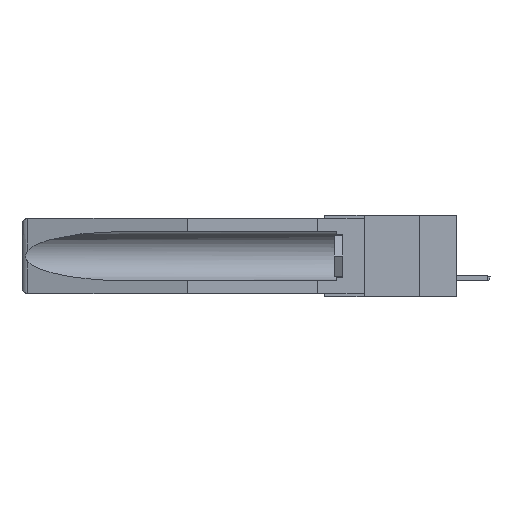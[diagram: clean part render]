
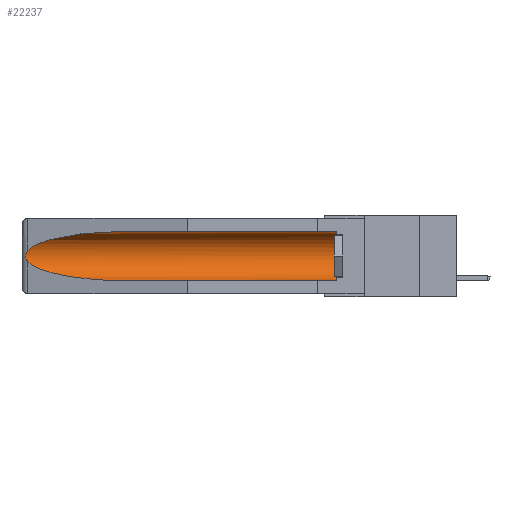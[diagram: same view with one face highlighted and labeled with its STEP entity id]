
A CAD part, left-side view. The second image highlights one B-rep face of the part: STEP entity #22237.
In plain terms, the highlighted cylindrical face has radius 2.857 mm (diameter 5.715 mm), a partial arc.
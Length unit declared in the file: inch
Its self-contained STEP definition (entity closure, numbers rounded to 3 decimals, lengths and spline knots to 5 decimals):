
#723 = CARTESIAN_POINT ( 'NONE',  ( 0.26654, 1.53092, -0.15636 ) ) ;
#850 = ORIENTED_EDGE ( 'NONE', *, *, #21930, .T. ) ;
#1276 = CARTESIAN_POINT ( 'NONE',  ( 0.26597, 1.5296, -0.19026 ) ) ;
#1510 = FACE_OUTER_BOUND ( 'NONE', #3524, .T. ) ;
#1536 = VECTOR ( 'NONE', #4677, 39.37008 ) ;
#1788 = CARTESIAN_POINT ( 'NONE',  ( 0.2675, 1.53308, -0.17534 ) ) ;
#2054 = LINE ( 'NONE', #13014, #4106 ) ;
#3070 = B_SPLINE_CURVE_WITH_KNOTS ( 'NONE', 3,
 ( #3275, #9907, #723, #17129, #3477, #1788, #18815, #14418, #1276, #5667 ),
 .UNSPECIFIED., .F., .F.,
 ( 4, 2, 2, 2, 4 ),
 ( 0., 0.00029, 0.00058, 0.00087, 0.00117 ),
 .UNSPECIFIED. ) ;
#3275 = CARTESIAN_POINT ( 'NONE',  ( 0.26537, 1.52718, -0.14972 ) ) ;
#3477 = CARTESIAN_POINT ( 'NONE',  ( 0.2675, 1.53308, -0.16763 ) ) ;
#3524 = EDGE_LOOP ( 'NONE', ( #13509, #11887, #20888, #19044, #21107, #850 ) ) ;
#4014 = CARTESIAN_POINT ( 'NONE',  ( 0.155, 1.07973, -0.059 ) ) ;
#4043 = VERTEX_POINT ( 'NONE', #14770 ) ;
#4106 = VECTOR ( 'NONE', #6475, 39.37008 ) ;
#4454 = CARTESIAN_POINT ( 'NONE',  ( 0.25451, 1.48313, -0.24835 ) ) ;
#4677 = DIRECTION ( 'NONE',  ( 0., 1., 0. ) ) ;
#5005 =( BOUNDED_CURVE ( )  B_SPLINE_CURVE ( 3, ( #15228, #4454, #21779, #19602 ),
 .UNSPECIFIED., .F., .F. ) 
 B_SPLINE_CURVE_WITH_KNOTS ( ( 4, 4 ),
 ( 0.1948, 1.5708 ),
 .UNSPECIFIED. ) 
 CURVE ( )  GEOMETRIC_REPRESENTATION_ITEM ( )  RATIONAL_B_SPLINE_CURVE ( ( 1., 0.848, 0.848, 1. ) ) 
 REPRESENTATION_ITEM ( '' )  );
#5667 = CARTESIAN_POINT ( 'NONE',  ( 0.26537, 1.52718, -0.19328 ) ) ;
#6019 = CARTESIAN_POINT ( 'NONE',  ( 0.25451, 1.48313, -0.09465 ) ) ;
#6438 = EDGE_CURVE ( 'NONE', #26772, #28308, #10365, .T. ) ;
#6475 = DIRECTION ( 'NONE',  ( 0., 1., 0. ) ) ;
#7294 = CARTESIAN_POINT ( 'NONE',  ( 0.155, 0.126, -0.284 ) ) ;
#7404 = EDGE_CURVE ( 'NONE', #4043, #26897, #5005, .T. ) ;
#7608 = CARTESIAN_POINT ( 'NONE',  ( 0.155, 1.07973, -0.059 ) ) ;
#8822 = VERTEX_POINT ( 'NONE', #18067 ) ;
#9035 =( BOUNDED_CURVE ( )  B_SPLINE_CURVE ( 3, ( #4014, #17262, #6019, #19063 ),
 .UNSPECIFIED., .F., .F. ) 
 B_SPLINE_CURVE_WITH_KNOTS ( ( 4, 4 ),
 ( 4.71239, 6.08839 ),
 .UNSPECIFIED. ) 
 CURVE ( )  GEOMETRIC_REPRESENTATION_ITEM ( )  RATIONAL_B_SPLINE_CURVE ( ( 1., 0.848, 0.848, 1. ) ) 
 REPRESENTATION_ITEM ( '' )  );
#9907 = CARTESIAN_POINT ( 'NONE',  ( 0.26597, 1.52961, -0.15275 ) ) ;
#10365 = CIRCLE ( 'NONE', #13284, 0.1125 ) ;
#11305 = EDGE_CURVE ( 'NONE', #26772, #26897, #2054, .T. ) ;
#11887 = ORIENTED_EDGE ( 'NONE', *, *, #16082, .T. ) ;
#13014 = CARTESIAN_POINT ( 'NONE',  ( 0.155, -0.30754, -0.284 ) ) ;
#13284 = AXIS2_PLACEMENT_3D ( 'NONE', #22628, #14039, #27273 ) ;
#13509 = ORIENTED_EDGE ( 'NONE', *, *, #24779, .T. ) ;
#14039 = DIRECTION ( 'NONE',  ( 0., -1., 0. ) ) ;
#14418 = CARTESIAN_POINT ( 'NONE',  ( 0.26655, 1.53094, -0.18657 ) ) ;
#14447 = CARTESIAN_POINT ( 'NONE',  ( 0.155, -0.30754, -0.1715 ) ) ;
#14770 = CARTESIAN_POINT ( 'NONE',  ( 0.26537, 1.52718, -0.19328 ) ) ;
#15228 = CARTESIAN_POINT ( 'NONE',  ( 0.26537, 1.52718, -0.19328 ) ) ;
#15832 = CARTESIAN_POINT ( 'NONE',  ( 0.155, -0.30754, -0.059 ) ) ;
#16082 = EDGE_CURVE ( 'NONE', #8822, #4043, #3070, .T. ) ;
#16663 = DIRECTION ( 'NONE',  ( 0., 1., 0. ) ) ;
#17129 = CARTESIAN_POINT ( 'NONE',  ( 0.2673, 1.5327, -0.16383 ) ) ;
#17262 = CARTESIAN_POINT ( 'NONE',  ( 0.21114, 1.30732, -0.059 ) ) ;
#18067 = CARTESIAN_POINT ( 'NONE',  ( 0.26537, 1.52718, -0.14972 ) ) ;
#18815 = CARTESIAN_POINT ( 'NONE',  ( 0.2673, 1.53269, -0.17917 ) ) ;
#19044 = ORIENTED_EDGE ( 'NONE', *, *, #11305, .F. ) ;
#19063 = CARTESIAN_POINT ( 'NONE',  ( 0.26537, 1.52718, -0.14972 ) ) ;
#19602 = CARTESIAN_POINT ( 'NONE',  ( 0.155, 1.07973, -0.284 ) ) ;
#20888 = ORIENTED_EDGE ( 'NONE', *, *, #7404, .T. ) ;
#21107 = ORIENTED_EDGE ( 'NONE', *, *, #6438, .T. ) ;
#21546 = CARTESIAN_POINT ( 'NONE',  ( 0.155, 0.126, -0.059 ) ) ;
#21737 = CYLINDRICAL_SURFACE ( 'NONE', #22564, 0.1125 ) ;
#21779 = CARTESIAN_POINT ( 'NONE',  ( 0.21114, 1.30732, -0.284 ) ) ;
#21930 = EDGE_CURVE ( 'NONE', #28308, #25965, #22759, .T. ) ;
#22237 = ADVANCED_FACE ( 'NONE', ( #1510 ), #21737, .F. ) ;
#22564 = AXIS2_PLACEMENT_3D ( 'NONE', #14447, #16663, #27397 ) ;
#22628 = CARTESIAN_POINT ( 'NONE',  ( 0.155, 0.126, -0.1715 ) ) ;
#22759 = LINE ( 'NONE', #15832, #1536 ) ;
#23153 = CARTESIAN_POINT ( 'NONE',  ( 0.155, 1.07973, -0.284 ) ) ;
#24779 = EDGE_CURVE ( 'NONE', #25965, #8822, #9035, .T. ) ;
#25965 = VERTEX_POINT ( 'NONE', #7608 ) ;
#26772 = VERTEX_POINT ( 'NONE', #7294 ) ;
#26897 = VERTEX_POINT ( 'NONE', #23153 ) ;
#27273 = DIRECTION ( 'NONE',  ( 0., 0., 1. ) ) ;
#27397 = DIRECTION ( 'NONE',  ( 0., 0., 1. ) ) ;
#28308 = VERTEX_POINT ( 'NONE', #21546 ) ;
